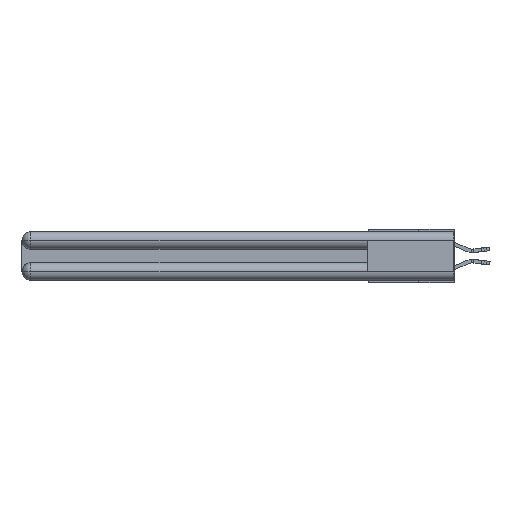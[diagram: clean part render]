
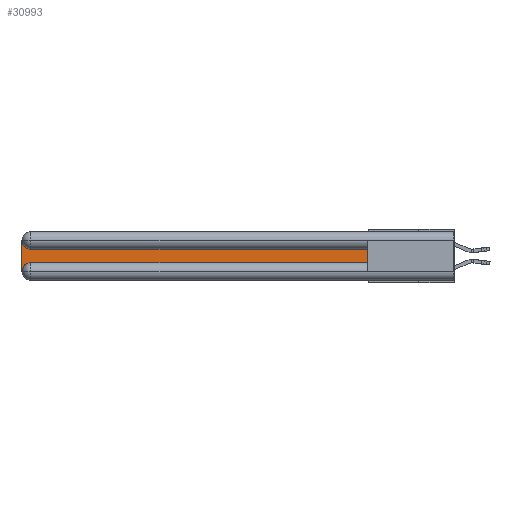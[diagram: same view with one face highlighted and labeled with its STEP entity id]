
A CAD part, left-side view. The second image highlights one B-rep face of the part: STEP entity #30993.
In plain terms, the highlighted planar face has unit normal (-1, 0, 0).
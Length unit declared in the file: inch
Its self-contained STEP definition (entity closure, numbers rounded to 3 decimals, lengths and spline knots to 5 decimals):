
#1083 = CARTESIAN_POINT ( 'NONE',  ( 0.075, 0.6, -0.2175 ) ) ;
#1865 = DIRECTION ( 'NONE',  ( 0., 1., 0. ) ) ;
#2249 = LINE ( 'NONE', #1083, #30740 ) ;
#2288 = ORIENTED_EDGE ( 'NONE', *, *, #27510, .T. ) ;
#2836 = VERTEX_POINT ( 'NONE', #9542 ) ;
#3650 = CARTESIAN_POINT ( 'NONE',  ( 0.075, 2.94, -0.2175 ) ) ;
#3722 = EDGE_CURVE ( 'NONE', #15094, #22788, #23970, .T. ) ;
#4715 = DIRECTION ( 'NONE',  ( 1., 0., 0. ) ) ;
#5737 = DIRECTION ( 'NONE',  ( 1., 0., 0. ) ) ;
#8405 = CIRCLE ( 'NONE', #17111, 0.06 ) ;
#8556 = AXIS2_PLACEMENT_3D ( 'NONE', #10337, #5737, #25503 ) ;
#9519 = CARTESIAN_POINT ( 'NONE',  ( 0.075, 0.6, -0.1225 ) ) ;
#9542 = CARTESIAN_POINT ( 'NONE',  ( 0.075, 0.6, -0.1225 ) ) ;
#9636 = ORIENTED_EDGE ( 'NONE', *, *, #31701, .T. ) ;
#10337 = CARTESIAN_POINT ( 'NONE',  ( 0.075, 3., -0.1225 ) ) ;
#10389 = CIRCLE ( 'NONE', #29217, 0.06 ) ;
#10457 = EDGE_LOOP ( 'NONE', ( #16510, #30859, #15264, #2288, #9636, #16602 ) ) ;
#11100 = DIRECTION ( 'NONE',  ( 0., 0., 1. ) ) ;
#12120 = EDGE_CURVE ( 'NONE', #12424, #2836, #2249, .T. ) ;
#12424 = VERTEX_POINT ( 'NONE', #21312 ) ;
#12576 = VECTOR ( 'NONE', #19214, 39.37008 ) ;
#12898 = CARTESIAN_POINT ( 'NONE',  ( 0.075, 3., -0.2175 ) ) ;
#12921 = EDGE_CURVE ( 'NONE', #2836, #14250, #22965, .T. ) ;
#14250 = VERTEX_POINT ( 'NONE', #15803 ) ;
#15094 = VERTEX_POINT ( 'NONE', #31244 ) ;
#15264 = ORIENTED_EDGE ( 'NONE', *, *, #3722, .T. ) ;
#15803 = CARTESIAN_POINT ( 'NONE',  ( 0.075, 2.94, -0.1225 ) ) ;
#16510 = ORIENTED_EDGE ( 'NONE', *, *, #12921, .T. ) ;
#16602 = ORIENTED_EDGE ( 'NONE', *, *, #12120, .T. ) ;
#16832 = CARTESIAN_POINT ( 'NONE',  ( 0.075, 0.6, -0.2175 ) ) ;
#17111 = AXIS2_PLACEMENT_3D ( 'NONE', #17416, #4715, #20012 ) ;
#17416 = CARTESIAN_POINT ( 'NONE',  ( 0.075, 2.94, -0.2775 ) ) ;
#19214 = DIRECTION ( 'NONE',  ( 0., -1., 0. ) ) ;
#19215 = CARTESIAN_POINT ( 'NONE',  ( 0.075, 3., -0.2775 ) ) ;
#20012 = DIRECTION ( 'NONE',  ( 0., 0., -1. ) ) ;
#20196 = VERTEX_POINT ( 'NONE', #3650 ) ;
#20307 = PLANE ( 'NONE',  #8556 ) ;
#20640 = DIRECTION ( 'NONE',  ( 0., 0., -1. ) ) ;
#21312 = CARTESIAN_POINT ( 'NONE',  ( 0.075, 0.6, -0.2175 ) ) ;
#22788 = VERTEX_POINT ( 'NONE', #19215 ) ;
#22965 = LINE ( 'NONE', #9519, #32262 ) ;
#22985 = CARTESIAN_POINT ( 'NONE',  ( 0.075, 2.94, -0.0625 ) ) ;
#23214 = VECTOR ( 'NONE', #30459, 39.37008 ) ;
#23970 = LINE ( 'NONE', #12898, #23214 ) ;
#25223 = DIRECTION ( 'NONE',  ( 1., 0., 0. ) ) ;
#25503 = DIRECTION ( 'NONE',  ( 0., 0., -1. ) ) ;
#26701 = FACE_OUTER_BOUND ( 'NONE', #10457, .T. ) ;
#27510 = EDGE_CURVE ( 'NONE', #22788, #20196, #8405, .T. ) ;
#28650 = EDGE_CURVE ( 'NONE', #14250, #15094, #10389, .T. ) ;
#28992 = LINE ( 'NONE', #16832, #12576 ) ;
#29217 = AXIS2_PLACEMENT_3D ( 'NONE', #22985, #25223, #20640 ) ;
#30459 = DIRECTION ( 'NONE',  ( 0., 0., -1. ) ) ;
#30740 = VECTOR ( 'NONE', #11100, 39.37008 ) ;
#30859 = ORIENTED_EDGE ( 'NONE', *, *, #28650, .T. ) ;
#30993 = ADVANCED_FACE ( 'NONE', ( #26701 ), #20307, .F. ) ;
#31244 = CARTESIAN_POINT ( 'NONE',  ( 0.075, 3., -0.0625 ) ) ;
#31701 = EDGE_CURVE ( 'NONE', #20196, #12424, #28992, .T. ) ;
#32262 = VECTOR ( 'NONE', #1865, 39.37008 ) ;
